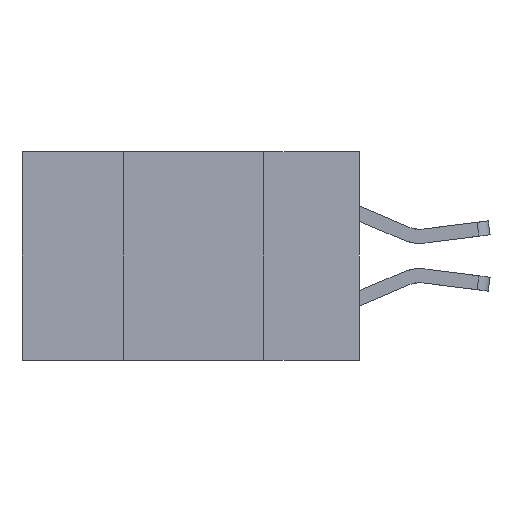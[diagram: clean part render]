
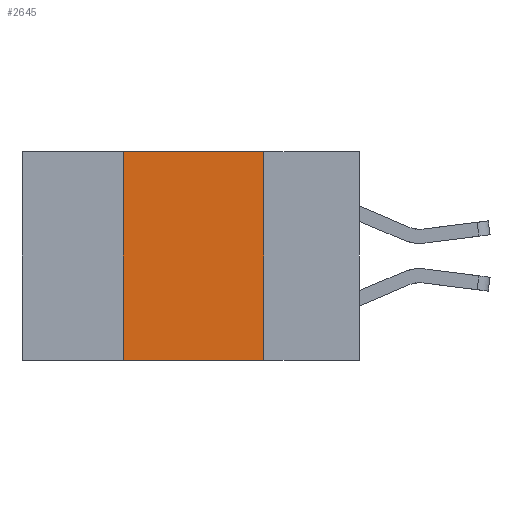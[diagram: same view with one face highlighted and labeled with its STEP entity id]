
A CAD part, left-side view. The second image highlights one B-rep face of the part: STEP entity #2645.
In plain terms, the highlighted planar face has unit normal (-1, 0, 0).
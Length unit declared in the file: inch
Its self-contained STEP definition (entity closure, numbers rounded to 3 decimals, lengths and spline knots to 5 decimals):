
#7 = CARTESIAN_POINT ( 'NONE',  ( 0., 0.42, -0.37 ) ) ;
#47 = VECTOR ( 'NONE', #7382, 39.37008 ) ;
#86 = CARTESIAN_POINT ( 'NONE',  ( 0., 0.6, 0. ) ) ;
#388 = DIRECTION ( 'NONE',  ( 0., -1., 0. ) ) ;
#787 = VECTOR ( 'NONE', #9085, 39.37008 ) ;
#1031 = LINE ( 'NONE', #9204, #9928 ) ;
#1112 = EDGE_CURVE ( 'NONE', #4106, #8895, #1031, .T. ) ;
#1296 = DIRECTION ( 'NONE',  ( 0., 0., -1. ) ) ;
#1325 = DIRECTION ( 'NONE',  ( 1., 0., 0. ) ) ;
#1396 = CARTESIAN_POINT ( 'NONE',  ( 0., 0.17, 0. ) ) ;
#1419 = AXIS2_PLACEMENT_3D ( 'NONE', #86, #1325, #1296 ) ;
#1991 = ORIENTED_EDGE ( 'NONE', *, *, #10109, .T. ) ;
#2288 = CARTESIAN_POINT ( 'NONE',  ( 0., 0.6, -0.37 ) ) ;
#2645 = ADVANCED_FACE ( 'NONE', ( #5579 ), #7440, .F. ) ;
#3205 = EDGE_LOOP ( 'NONE', ( #8216, #10116, #5373, #1991 ) ) ;
#3947 = VECTOR ( 'NONE', #388, 39.37008 ) ;
#4106 = VERTEX_POINT ( 'NONE', #6797 ) ;
#5127 = LINE ( 'NONE', #10658, #47 ) ;
#5280 = EDGE_CURVE ( 'NONE', #8895, #7299, #5515, .T. ) ;
#5373 = ORIENTED_EDGE ( 'NONE', *, *, #10653, .F. ) ;
#5515 = LINE ( 'NONE', #1396, #787 ) ;
#5579 = FACE_OUTER_BOUND ( 'NONE', #3205, .T. ) ;
#6068 = CARTESIAN_POINT ( 'NONE',  ( 0., 0.17, 0. ) ) ;
#6797 = CARTESIAN_POINT ( 'NONE',  ( 0., 0.42, 0. ) ) ;
#7299 = VERTEX_POINT ( 'NONE', #9015 ) ;
#7382 = DIRECTION ( 'NONE',  ( 0., 0., 1. ) ) ;
#7440 = PLANE ( 'NONE',  #1419 ) ;
#8216 = ORIENTED_EDGE ( 'NONE', *, *, #5280, .F. ) ;
#8753 = LINE ( 'NONE', #2288, #3947 ) ;
#8895 = VERTEX_POINT ( 'NONE', #6068 ) ;
#9015 = CARTESIAN_POINT ( 'NONE',  ( 0., 0.17, -0.37 ) ) ;
#9085 = DIRECTION ( 'NONE',  ( 0., 0., -1. ) ) ;
#9204 = CARTESIAN_POINT ( 'NONE',  ( 0., 0.6, 0. ) ) ;
#9541 = DIRECTION ( 'NONE',  ( 0., -1., 0. ) ) ;
#9606 = VERTEX_POINT ( 'NONE', #7 ) ;
#9928 = VECTOR ( 'NONE', #9541, 39.37008 ) ;
#10109 = EDGE_CURVE ( 'NONE', #9606, #7299, #8753, .T. ) ;
#10116 = ORIENTED_EDGE ( 'NONE', *, *, #1112, .F. ) ;
#10653 = EDGE_CURVE ( 'NONE', #9606, #4106, #5127, .T. ) ;
#10658 = CARTESIAN_POINT ( 'NONE',  ( 0., 0.42, 0. ) ) ;
